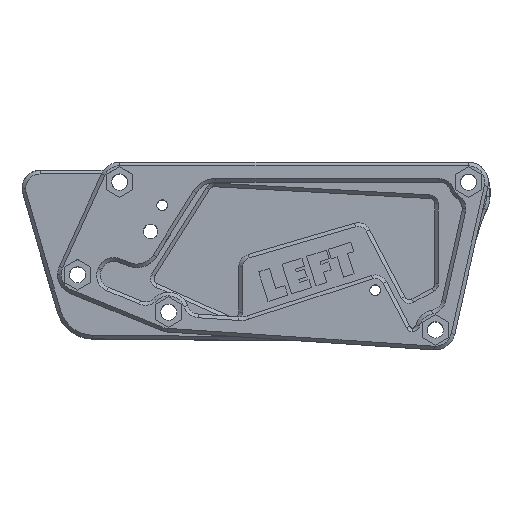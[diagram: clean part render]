
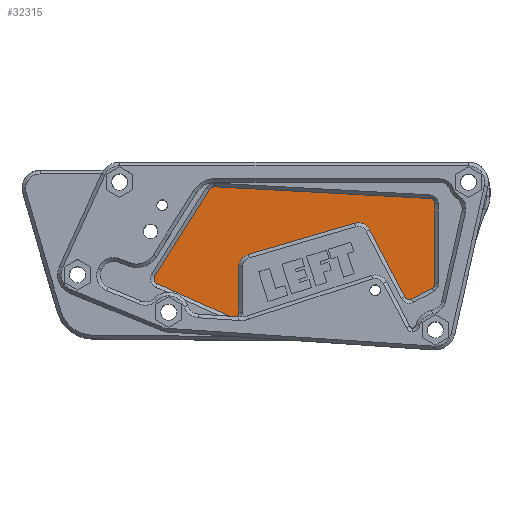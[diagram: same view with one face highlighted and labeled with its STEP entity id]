
A CAD part, top view. The second image highlights one B-rep face of the part: STEP entity #32315.
In plain terms, the highlighted planar face has unit normal (0, 0, 1).
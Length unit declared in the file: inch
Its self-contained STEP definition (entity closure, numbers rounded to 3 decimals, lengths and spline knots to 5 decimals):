
#497 = CARTESIAN_POINT ( 'NONE',  ( 3.67252, 0.3845, 1.25417 ) ) ;
#1331 = CARTESIAN_POINT ( 'NONE',  ( 2.09516, 0.9197, 1.25417 ) ) ;
#1334 = CARTESIAN_POINT ( 'NONE',  ( 4.51489, 0.73086, 1.25417 ) ) ;
#1539 = DIRECTION ( 'NONE',  ( -1., 0., 0. ) ) ;
#2223 = EDGE_CURVE ( 'NONE', #21261, #20757, #8957, .T. ) ;
#2322 = CARTESIAN_POINT ( 'NONE',  ( 2.36297, -0.45607, 1.25417 ) ) ;
#2367 = ORIENTED_EDGE ( 'NONE', *, *, #9406, .T. ) ;
#2491 = PLANE ( 'NONE',  #5284 ) ;
#2894 = VERTEX_POINT ( 'NONE', #21141 ) ;
#2937 = AXIS2_PLACEMENT_3D ( 'NONE', #497, #6786, #3432 ) ;
#3432 = DIRECTION ( 'NONE',  ( -1., 0., 0. ) ) ;
#3798 = EDGE_CURVE ( 'NONE', #7035, #13341, #22994, .T. ) ;
#4172 = CARTESIAN_POINT ( 'NONE',  ( 4.1827, -0.2873, 1.25417 ) ) ;
#4379 = LINE ( 'NONE', #26960, #31168 ) ;
#4719 = DIRECTION ( 'NONE',  ( 0., 0., 1. ) ) ;
#4736 = DIRECTION ( 'NONE',  ( 0., 0., 1. ) ) ;
#5031 = CARTESIAN_POINT ( 'NONE',  ( 4.51489, 0.73086, 1.25417 ) ) ;
#5284 = AXIS2_PLACEMENT_3D ( 'NONE', #5852, #38038, #40339 ) ;
#5852 = CARTESIAN_POINT ( 'NONE',  ( 0., 0., 1.25417 ) ) ;
#6305 = AXIS2_PLACEMENT_3D ( 'NONE', #33179, #39619, #10761 ) ;
#6786 = DIRECTION ( 'NONE',  ( 0., 0., -1. ) ) ;
#7035 = VERTEX_POINT ( 'NONE', #15810 ) ;
#7090 = CIRCLE ( 'NONE', #8406, 0.06 ) ;
#7407 = DIRECTION ( 'NONE',  ( -0.999, 0.054, 0. ) ) ;
#7421 = CARTESIAN_POINT ( 'NONE',  ( 4.51489, -0.14464, 1.25417 ) ) ;
#7489 = VERTEX_POINT ( 'NONE', #5031 ) ;
#7584 = CIRCLE ( 'NONE', #28302, 0.06 ) ;
#7755 = CARTESIAN_POINT ( 'NONE',  ( 4.1827, -0.2873, 1.25417 ) ) ;
#8285 = CARTESIAN_POINT ( 'NONE',  ( 4.45815, 0.79077, 1.25417 ) ) ;
#8406 = AXIS2_PLACEMENT_3D ( 'NONE', #23492, #17419, #1539 ) ;
#8574 = VECTOR ( 'NONE', #29704, 39.37008 ) ;
#8957 = CIRCLE ( 'NONE', #32360, 0.06 ) ;
#9406 = EDGE_CURVE ( 'NONE', #13341, #17606, #12019, .T. ) ;
#9443 = EDGE_CURVE ( 'NONE', #16073, #16214, #28549, .T. ) ;
#10008 = EDGE_CURVE ( 'NONE', #7489, #27699, #16960, .T. ) ;
#10098 = ORIENTED_EDGE ( 'NONE', *, *, #35535, .T. ) ;
#10761 = DIRECTION ( 'NONE',  ( -1., 0., 0. ) ) ;
#10967 = AXIS2_PLACEMENT_3D ( 'NONE', #17651, #4719, #30446 ) ;
#11058 = EDGE_CURVE ( 'NONE', #18646, #2894, #22945, .T. ) ;
#11153 = LINE ( 'NONE', #1334, #18441 ) ;
#11216 = ORIENTED_EDGE ( 'NONE', *, *, #13867, .T. ) ;
#11342 = EDGE_CURVE ( 'NONE', #17606, #27772, #14962, .T. ) ;
#11438 = CARTESIAN_POINT ( 'NONE',  ( 1.44201, -0.05951, 1.25417 ) ) ;
#11523 = VERTEX_POINT ( 'NONE', #7755 ) ;
#11605 = CARTESIAN_POINT ( 'NONE',  ( 1.44201, -0.05951, 1.25417 ) ) ;
#12003 = LINE ( 'NONE', #21011, #23060 ) ;
#12019 = LINE ( 'NONE', #11605, #15623 ) ;
#12158 = DIRECTION ( 'NONE',  ( 0., 0., 1. ) ) ;
#12335 = EDGE_CURVE ( 'NONE', #33068, #16073, #7584, .T. ) ;
#12825 = DIRECTION ( 'NONE',  ( 0., 1., 0. ) ) ;
#13234 = ORIENTED_EDGE ( 'NONE', *, *, #11058, .T. ) ;
#13341 = VERTEX_POINT ( 'NONE', #29349 ) ;
#13421 = ORIENTED_EDGE ( 'NONE', *, *, #11342, .T. ) ;
#13867 = EDGE_CURVE ( 'NONE', #2894, #11523, #24240, .T. ) ;
#14755 = ORIENTED_EDGE ( 'NONE', *, *, #9443, .T. ) ;
#14962 = CIRCLE ( 'NONE', #38331, 0.06 ) ;
#15096 = CARTESIAN_POINT ( 'NONE',  ( 1.49277, -0.09148, 1.25417 ) ) ;
#15522 = VERTEX_POINT ( 'NONE', #22381 ) ;
#15550 = EDGE_CURVE ( 'NONE', #32093, #18646, #12003, .T. ) ;
#15623 = VECTOR ( 'NONE', #40854, 39.37008 ) ;
#15663 = CARTESIAN_POINT ( 'NONE',  ( 2.50297, 0.043, 1.25417 ) ) ;
#15810 = CARTESIAN_POINT ( 'NONE',  ( 2.09516, 0.9197, 1.25417 ) ) ;
#16073 = VERTEX_POINT ( 'NONE', #2322 ) ;
#16163 = CARTESIAN_POINT ( 'NONE',  ( 2.36297, 0.043, 1.25417 ) ) ;
#16212 = EDGE_CURVE ( 'NONE', #27772, #33068, #4379, .T. ) ;
#16214 = VERTEX_POINT ( 'NONE', #30532 ) ;
#16960 = CIRCLE ( 'NONE', #10967, 0.06 ) ;
#17344 = VECTOR ( 'NONE', #7407, 39.37008 ) ;
#17419 = DIRECTION ( 'NONE',  ( 0., 0., 1. ) ) ;
#17606 = VERTEX_POINT ( 'NONE', #11438 ) ;
#17651 = CARTESIAN_POINT ( 'NONE',  ( 4.45489, 0.73086, 1.25417 ) ) ;
#18441 = VECTOR ( 'NONE', #30205, 39.37008 ) ;
#18626 = LINE ( 'NONE', #40392, #29183 ) ;
#18646 = VERTEX_POINT ( 'NONE', #26525 ) ;
#19049 = DIRECTION ( 'NONE',  ( -1., 0., 0. ) ) ;
#19801 = EDGE_CURVE ( 'NONE', #11523, #15522, #7090, .T. ) ;
#20757 = VERTEX_POINT ( 'NONE', #7421 ) ;
#21011 = CARTESIAN_POINT ( 'NONE',  ( 3.63328, 0.51889, 1.25417 ) ) ;
#21141 = CARTESIAN_POINT ( 'NONE',  ( 3.79652, 0.4495, 1.25417 ) ) ;
#21261 = VERTEX_POINT ( 'NONE', #27242 ) ;
#21277 = EDGE_CURVE ( 'NONE', #15522, #21261, #18626, .T. ) ;
#21768 = ORIENTED_EDGE ( 'NONE', *, *, #12335, .T. ) ;
#21853 = ORIENTED_EDGE ( 'NONE', *, *, #39348, .T. ) ;
#22021 = CARTESIAN_POINT ( 'NONE',  ( 2.46373, 0.17738, 1.25417 ) ) ;
#22381 = CARTESIAN_POINT ( 'NONE',  ( 4.2637, -0.31259, 1.25417 ) ) ;
#22945 = CIRCLE ( 'NONE', #2937, 0.14 ) ;
#22994 = CIRCLE ( 'NONE', #6305, 0.06 ) ;
#23060 = VECTOR ( 'NONE', #33782, 39.37008 ) ;
#23492 = CARTESIAN_POINT ( 'NONE',  ( 4.23584, -0.25945, 1.25417 ) ) ;
#24240 = LINE ( 'NONE', #4172, #8574 ) ;
#24928 = DIRECTION ( 'NONE',  ( 0., 0., 1. ) ) ;
#25124 = ORIENTED_EDGE ( 'NONE', *, *, #10008, .T. ) ;
#25299 = DIRECTION ( 'NONE',  ( -1., 0., 0. ) ) ;
#25379 = EDGE_CURVE ( 'NONE', #16214, #32093, #31441, .T. ) ;
#26525 = CARTESIAN_POINT ( 'NONE',  ( 3.63328, 0.51889, 1.25417 ) ) ;
#26960 = CARTESIAN_POINT ( 'NONE',  ( 2.27835, -0.51079, 1.25417 ) ) ;
#27242 = CARTESIAN_POINT ( 'NONE',  ( 4.48274, -0.19778, 1.25417 ) ) ;
#27471 = ORIENTED_EDGE ( 'NONE', *, *, #15550, .T. ) ;
#27699 = VERTEX_POINT ( 'NONE', #8285 ) ;
#27772 = VERTEX_POINT ( 'NONE', #31090 ) ;
#27870 = DIRECTION ( 'NONE',  ( -1., 0., 0. ) ) ;
#28302 = AXIS2_PLACEMENT_3D ( 'NONE', #28497, #24928, #19049 ) ;
#28420 = FACE_OUTER_BOUND ( 'NONE', #31745, .T. ) ;
#28497 = CARTESIAN_POINT ( 'NONE',  ( 2.30297, -0.45607, 1.25417 ) ) ;
#28549 = LINE ( 'NONE', #16163, #40322 ) ;
#29183 = VECTOR ( 'NONE', #37267, 39.37008 ) ;
#29223 = CARTESIAN_POINT ( 'NONE',  ( 4.45489, -0.14464, 1.25417 ) ) ;
#29349 = CARTESIAN_POINT ( 'NONE',  ( 2.04112, 0.89176, 1.25417 ) ) ;
#29516 = ORIENTED_EDGE ( 'NONE', *, *, #21277, .T. ) ;
#29534 = ORIENTED_EDGE ( 'NONE', *, *, #16212, .T. ) ;
#29704 = DIRECTION ( 'NONE',  ( 0.464, -0.886, 0. ) ) ;
#30028 = ORIENTED_EDGE ( 'NONE', *, *, #19801, .T. ) ;
#30205 = DIRECTION ( 'NONE',  ( 0., 1., 0. ) ) ;
#30446 = DIRECTION ( 'NONE',  ( -1., 0., 0. ) ) ;
#30532 = CARTESIAN_POINT ( 'NONE',  ( 2.36297, 0.043, 1.25417 ) ) ;
#31090 = CARTESIAN_POINT ( 'NONE',  ( 1.46815, -0.1462, 1.25417 ) ) ;
#31168 = VECTOR ( 'NONE', #33880, 39.37008 ) ;
#31441 = CIRCLE ( 'NONE', #39405, 0.14 ) ;
#31745 = EDGE_LOOP ( 'NONE', ( #13234, #11216, #30028, #29516, #39213, #21853, #25124, #10098, #34279, #2367, #13421, #29534, #21768, #14755, #39060, #27471 ) ) ;
#32093 = VERTEX_POINT ( 'NONE', #22021 ) ;
#32315 = ADVANCED_FACE ( 'NONE', ( #28420 ), #2491, .F. ) ;
#32360 = AXIS2_PLACEMENT_3D ( 'NONE', #29223, #4736, #36921 ) ;
#33068 = VERTEX_POINT ( 'NONE', #37321 ) ;
#33179 = CARTESIAN_POINT ( 'NONE',  ( 2.09189, 0.85979, 1.25417 ) ) ;
#33782 = DIRECTION ( 'NONE',  ( 0.96, 0.28, 0. ) ) ;
#33880 = DIRECTION ( 'NONE',  ( 0.912, -0.41, 0. ) ) ;
#34279 = ORIENTED_EDGE ( 'NONE', *, *, #3798, .T. ) ;
#35126 = DIRECTION ( 'NONE',  ( 0., 0., -1. ) ) ;
#35535 = EDGE_CURVE ( 'NONE', #27699, #7035, #36059, .T. ) ;
#36059 = LINE ( 'NONE', #1331, #17344 ) ;
#36921 = DIRECTION ( 'NONE',  ( -1., 0., 0. ) ) ;
#37267 = DIRECTION ( 'NONE',  ( 0.886, 0.464, 0. ) ) ;
#37321 = CARTESIAN_POINT ( 'NONE',  ( 2.27835, -0.51079, 1.25417 ) ) ;
#38038 = DIRECTION ( 'NONE',  ( 0., 0., -1. ) ) ;
#38331 = AXIS2_PLACEMENT_3D ( 'NONE', #15096, #12158, #27870 ) ;
#39060 = ORIENTED_EDGE ( 'NONE', *, *, #25379, .T. ) ;
#39213 = ORIENTED_EDGE ( 'NONE', *, *, #2223, .T. ) ;
#39348 = EDGE_CURVE ( 'NONE', #20757, #7489, #11153, .T. ) ;
#39405 = AXIS2_PLACEMENT_3D ( 'NONE', #15663, #35126, #25299 ) ;
#39619 = DIRECTION ( 'NONE',  ( 0., 0., 1. ) ) ;
#40322 = VECTOR ( 'NONE', #12825, 39.37008 ) ;
#40339 = DIRECTION ( 'NONE',  ( -1., 0., 0. ) ) ;
#40392 = CARTESIAN_POINT ( 'NONE',  ( 4.48274, -0.19778, 1.25417 ) ) ;
#40854 = DIRECTION ( 'NONE',  ( -0.533, -0.846, 0. ) ) ;
